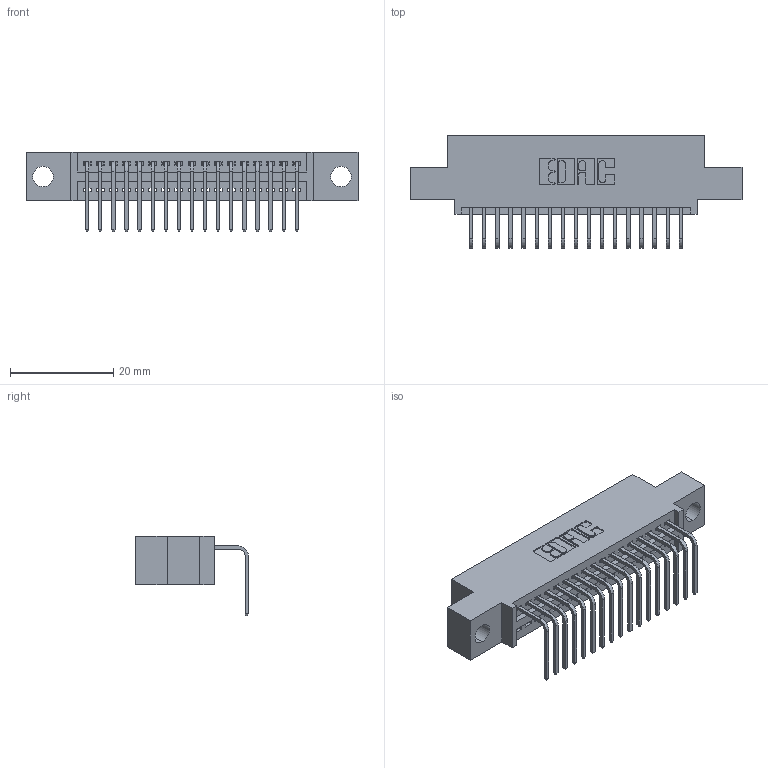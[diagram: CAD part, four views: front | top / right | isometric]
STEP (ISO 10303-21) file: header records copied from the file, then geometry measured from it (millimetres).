
FILE_DESCRIPTION (( 'STEP AP203' ), '1' );
FILE_NAME ('345-017-558-404.STEP', '2021-06-01T16:21:40', ( '' ), ( '' ), 'SwSTEP 2.0', 'SolidWorks 2020', '' );
FILE_SCHEMA (( 'CONFIG_CONTROL_DESIGN' ));
Length unit declared in the file: inch
Products named in the file (3): 345 Part_0.110 Offset - 0.156 Dia-TI; 345-017-558-404; 345-292-001_558 Tail - 2
Assembly tree (18 placements, depth 2):
  345-017-558-404
    345 Part_0.110 Offset - 0.156 Dia-TI
    345-292-001_558 Tail - 2  x17
Bounding box: 64.39 x 21.83 x 15.37 mm (x, y, z)
Volume: 5788.3 mm3; surface area: 7609.5 mm2
Topology: 18 solids, 18 shells, 1164 faces, 3483 edges, 2298 vertices
Faces by surface type: plane 812, cylinder 352
Entity records: 16795 total; most frequent: CARTESIAN_POINT 2921, ORIENTED_EDGE 2870, DIRECTION 2585, EDGE_CURVE 1435, VECTOR 1235, LINE 1235, VERTEX_POINT 954, AXIS2_PLACEMENT_3D 675
